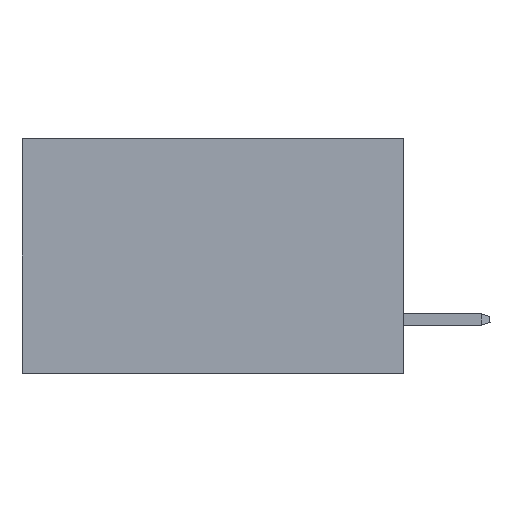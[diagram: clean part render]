
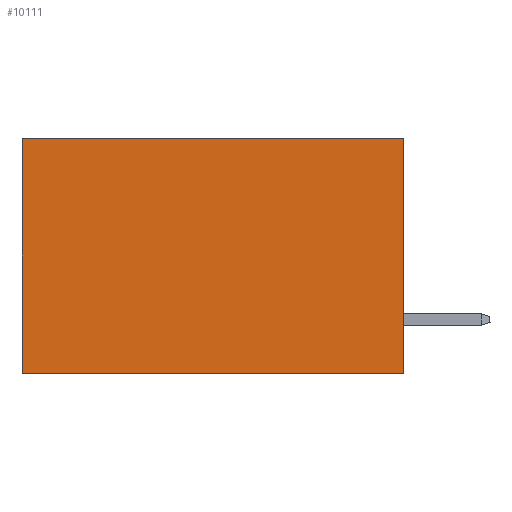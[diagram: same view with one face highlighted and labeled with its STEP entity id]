
A CAD part, left-side view. The second image highlights one B-rep face of the part: STEP entity #10111.
In plain terms, the highlighted planar face has unit normal (-1, 0, 0).
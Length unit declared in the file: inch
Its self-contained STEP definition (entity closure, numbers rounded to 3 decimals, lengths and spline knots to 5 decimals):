
#396 = DIRECTION ( 'NONE',  ( 0., 1., 0. ) ) ;
#1343 = ORIENTED_EDGE ( 'NONE', *, *, #38861, .F. ) ;
#1447 = DIRECTION ( 'NONE',  ( 0., 0., -1. ) ) ;
#1760 = LINE ( 'NONE', #47247, #25666 ) ;
#6320 = LINE ( 'NONE', #48517, #48089 ) ;
#9295 = DIRECTION ( 'NONE',  ( 1., 0., 0. ) ) ;
#10111 = ADVANCED_FACE ( 'NONE', ( #47943 ), #13581, .F. ) ;
#11296 = LINE ( 'NONE', #27441, #27892 ) ;
#11335 = LINE ( 'NONE', #34573, #38898 ) ;
#12037 = ORIENTED_EDGE ( 'NONE', *, *, #24591, .F. ) ;
#13581 = PLANE ( 'NONE',  #20231 ) ;
#13916 = DIRECTION ( 'NONE',  ( 0., 0., -1. ) ) ;
#15399 = ORIENTED_EDGE ( 'NONE', *, *, #17888, .T. ) ;
#16580 = VERTEX_POINT ( 'NONE', #24489 ) ;
#17188 = DIRECTION ( 'NONE',  ( 0., 0., -1. ) ) ;
#17397 = VERTEX_POINT ( 'NONE', #48051 ) ;
#17888 = EDGE_CURVE ( 'NONE', #16580, #17397, #1760, .T. ) ;
#20231 = AXIS2_PLACEMENT_3D ( 'NONE', #28239, #9295, #1447 ) ;
#24489 = CARTESIAN_POINT ( 'NONE',  ( 0.2875, 0.6, 0. ) ) ;
#24591 = EDGE_CURVE ( 'NONE', #27373, #17397, #11335, .T. ) ;
#25666 = VECTOR ( 'NONE', #17188, 39.37008 ) ;
#27373 = VERTEX_POINT ( 'NONE', #39896 ) ;
#27441 = CARTESIAN_POINT ( 'NONE',  ( 0.2875, 0., 0. ) ) ;
#27633 = EDGE_LOOP ( 'NONE', ( #15399, #12037, #1343, #44541 ) ) ;
#27892 = VECTOR ( 'NONE', #396, 39.37008 ) ;
#28239 = CARTESIAN_POINT ( 'NONE',  ( 0.2875, 0., 0. ) ) ;
#30772 = DIRECTION ( 'NONE',  ( 0., 1., 0. ) ) ;
#34573 = CARTESIAN_POINT ( 'NONE',  ( 0.2875, 0., -0.37 ) ) ;
#38193 = EDGE_CURVE ( 'NONE', #43706, #16580, #11296, .T. ) ;
#38861 = EDGE_CURVE ( 'NONE', #43706, #27373, #6320, .T. ) ;
#38898 = VECTOR ( 'NONE', #30772, 39.37008 ) ;
#39896 = CARTESIAN_POINT ( 'NONE',  ( 0.2875, 0., -0.37 ) ) ;
#43706 = VERTEX_POINT ( 'NONE', #49239 ) ;
#44541 = ORIENTED_EDGE ( 'NONE', *, *, #38193, .T. ) ;
#47247 = CARTESIAN_POINT ( 'NONE',  ( 0.2875, 0.6, 0. ) ) ;
#47943 = FACE_OUTER_BOUND ( 'NONE', #27633, .T. ) ;
#48051 = CARTESIAN_POINT ( 'NONE',  ( 0.2875, 0.6, -0.37 ) ) ;
#48089 = VECTOR ( 'NONE', #13916, 39.37008 ) ;
#48517 = CARTESIAN_POINT ( 'NONE',  ( 0.2875, 0., 0. ) ) ;
#49239 = CARTESIAN_POINT ( 'NONE',  ( 0.2875, 0., 0. ) ) ;
